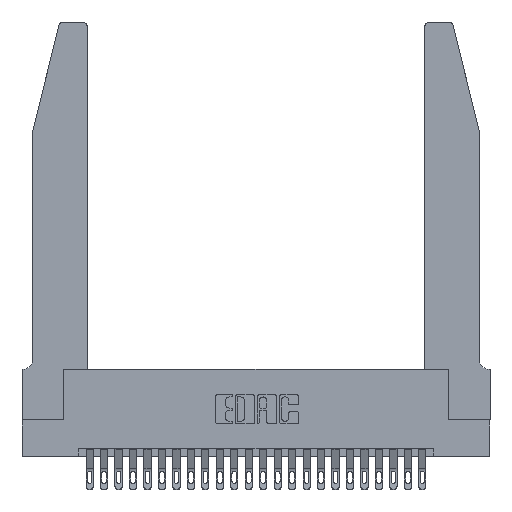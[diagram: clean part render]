
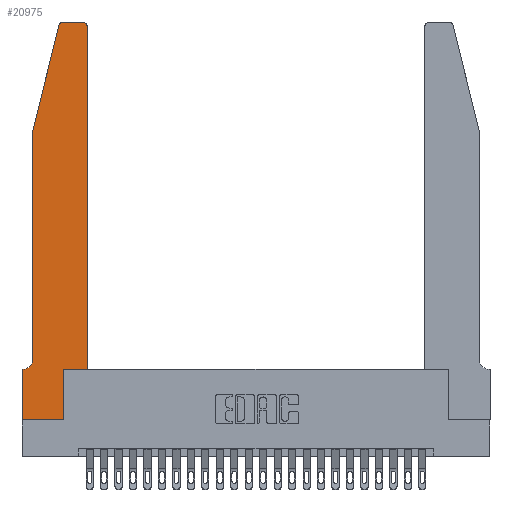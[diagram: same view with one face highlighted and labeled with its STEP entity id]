
A CAD part, top view. The second image highlights one B-rep face of the part: STEP entity #20975.
In plain terms, the highlighted planar face has unit normal (0, 0, 1).
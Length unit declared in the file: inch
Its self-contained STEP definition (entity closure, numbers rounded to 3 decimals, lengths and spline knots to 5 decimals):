
#20 = ORIENTED_EDGE ( 'NONE', *, *, #23290, .T. ) ;
#120 = CARTESIAN_POINT ( 'NONE',  ( 0.4505, 0.35, 0.37 ) ) ;
#456 = VECTOR ( 'NONE', #25401, 39.37008 ) ;
#581 = CARTESIAN_POINT ( 'NONE',  ( 0.4205, 2.72, 0.37 ) ) ;
#971 = DIRECTION ( 'NONE',  ( 0., -1., 0. ) ) ;
#1062 = VECTOR ( 'NONE', #4339, 39.37008 ) ;
#1375 = EDGE_LOOP ( 'NONE', ( #22535, #8584, #20704, #20, #17088, #1527, #10464, #9288, #26116, #14641, #14727, #2281 ) ) ;
#1527 = ORIENTED_EDGE ( 'NONE', *, *, #2855, .T. ) ;
#2210 = VECTOR ( 'NONE', #26248, 39.37008 ) ;
#2281 = ORIENTED_EDGE ( 'NONE', *, *, #10167, .T. ) ;
#2513 = CARTESIAN_POINT ( 'NONE',  ( 0., 0., 0.37 ) ) ;
#2573 = CARTESIAN_POINT ( 'NONE',  ( 0.4205, 2.75, 0.37 ) ) ;
#2686 = AXIS2_PLACEMENT_3D ( 'NONE', #581, #4804, #8976 ) ;
#2855 = EDGE_CURVE ( 'NONE', #21310, #16164, #23888, .T. ) ;
#3620 = CARTESIAN_POINT ( 'NONE',  ( 0.2605, 2.75, 0.37 ) ) ;
#4110 = DIRECTION ( 'NONE',  ( 0., 0., -1. ) ) ;
#4120 = DIRECTION ( 'NONE',  ( 0., 0., 1. ) ) ;
#4339 = DIRECTION ( 'NONE',  ( 1., 0., 0. ) ) ;
#4735 = PLANE ( 'NONE',  #20250 ) ;
#4804 = DIRECTION ( 'NONE',  ( 0., 0., 1. ) ) ;
#5156 = LINE ( 'NONE', #9257, #26128 ) ;
#6060 = VECTOR ( 'NONE', #12489, 39.37008 ) ;
#6342 = VERTEX_POINT ( 'NONE', #22943 ) ;
#6830 = CARTESIAN_POINT ( 'NONE',  ( 0.0055, 0.35, 0.37 ) ) ;
#6976 = DIRECTION ( 'NONE',  ( 0., -1., 0. ) ) ;
#7252 = CARTESIAN_POINT ( 'NONE',  ( 0.0755, 2., 0.37 ) ) ;
#7516 = CARTESIAN_POINT ( 'NONE',  ( 0.4505, 0.35, 0.37 ) ) ;
#7990 = VERTEX_POINT ( 'NONE', #2513 ) ;
#8584 = ORIENTED_EDGE ( 'NONE', *, *, #11825, .T. ) ;
#8708 = CIRCLE ( 'NONE', #20427, 0.07 ) ;
#8818 = VECTOR ( 'NONE', #17431, 39.37008 ) ;
#8968 = VERTEX_POINT ( 'NONE', #18181 ) ;
#8976 = DIRECTION ( 'NONE',  ( 1., 0., 0. ) ) ;
#9257 = CARTESIAN_POINT ( 'NONE',  ( 0.0755, 2., 0.37 ) ) ;
#9288 = ORIENTED_EDGE ( 'NONE', *, *, #12180, .T. ) ;
#9386 = FACE_OUTER_BOUND ( 'NONE', #1375, .T. ) ;
#9795 = DIRECTION ( 'NONE',  ( -1., 0., 0. ) ) ;
#9963 = LINE ( 'NONE', #120, #1062 ) ;
#10167 = EDGE_CURVE ( 'NONE', #8968, #24255, #17474, .T. ) ;
#10463 = VERTEX_POINT ( 'NONE', #10993 ) ;
#10464 = ORIENTED_EDGE ( 'NONE', *, *, #12732, .T. ) ;
#10773 = DIRECTION ( 'NONE',  ( 1., 0., 0. ) ) ;
#10993 = CARTESIAN_POINT ( 'NONE',  ( 0.4505, 0.35, 0.37 ) ) ;
#11049 = EDGE_CURVE ( 'NONE', #24833, #17696, #15502, .T. ) ;
#11497 = CARTESIAN_POINT ( 'NONE',  ( 0.0755, 2., 0.37 ) ) ;
#11825 = EDGE_CURVE ( 'NONE', #15092, #24833, #23747, .T. ) ;
#12180 = EDGE_CURVE ( 'NONE', #7990, #12327, #14835, .T. ) ;
#12327 = VERTEX_POINT ( 'NONE', #21972 ) ;
#12489 = DIRECTION ( 'NONE',  ( 0., 1., 0. ) ) ;
#12732 = EDGE_CURVE ( 'NONE', #16164, #7990, #16427, .T. ) ;
#13002 = CARTESIAN_POINT ( 'NONE',  ( 0., 0., 0.37 ) ) ;
#14641 = ORIENTED_EDGE ( 'NONE', *, *, #19251, .T. ) ;
#14671 = DIRECTION ( 'NONE',  ( 1., 0., 0. ) ) ;
#14727 = ORIENTED_EDGE ( 'NONE', *, *, #17780, .T. ) ;
#14788 = EDGE_CURVE ( 'NONE', #12327, #6342, #24489, .T. ) ;
#14835 = LINE ( 'NONE', #23316, #456 ) ;
#15092 = VERTEX_POINT ( 'NONE', #25351 ) ;
#15447 = VECTOR ( 'NONE', #9795, 39.37008 ) ;
#15502 = LINE ( 'NONE', #11497, #8818 ) ;
#15603 = CARTESIAN_POINT ( 'NONE',  ( 0.284, 2.72, 0.37 ) ) ;
#15745 = DIRECTION ( 'NONE',  ( 0., 1., 0. ) ) ;
#16164 = VERTEX_POINT ( 'NONE', #24701 ) ;
#16210 = AXIS2_PLACEMENT_3D ( 'NONE', #15603, #4120, #14671 ) ;
#16427 = LINE ( 'NONE', #13002, #24681 ) ;
#16743 = LINE ( 'NONE', #7516, #21543 ) ;
#16981 = CARTESIAN_POINT ( 'NONE',  ( 0.25487, 2.72718, 0.37 ) ) ;
#17088 = ORIENTED_EDGE ( 'NONE', *, *, #21775, .T. ) ;
#17431 = DIRECTION ( 'NONE',  ( -0.239, -0.971, 0. ) ) ;
#17474 = CIRCLE ( 'NONE', #2686, 0.03 ) ;
#17696 = VERTEX_POINT ( 'NONE', #7252 ) ;
#17780 = EDGE_CURVE ( 'NONE', #10463, #8968, #16743, .T. ) ;
#18181 = CARTESIAN_POINT ( 'NONE',  ( 0.4505, 2.72, 0.37 ) ) ;
#18197 = EDGE_CURVE ( 'NONE', #24255, #15092, #26252, .T. ) ;
#18326 = DIRECTION ( 'NONE',  ( -1., 0., 0. ) ) ;
#19251 = EDGE_CURVE ( 'NONE', #6342, #10463, #9963, .T. ) ;
#20009 = CARTESIAN_POINT ( 'NONE',  ( 0.0755, 0.42, 0.37 ) ) ;
#20250 = AXIS2_PLACEMENT_3D ( 'NONE', #20919, #23677, #10773 ) ;
#20298 = CARTESIAN_POINT ( 'NONE',  ( 0.0755, 0.35, 0.37 ) ) ;
#20427 = AXIS2_PLACEMENT_3D ( 'NONE', #22091, #4110, #18326 ) ;
#20704 = ORIENTED_EDGE ( 'NONE', *, *, #11049, .T. ) ;
#20919 = CARTESIAN_POINT ( 'NONE',  ( 0., 0.35, 0.37 ) ) ;
#20975 = ADVANCED_FACE ( 'NONE', ( #9386 ), #4735, .T. ) ;
#21310 = VERTEX_POINT ( 'NONE', #6830 ) ;
#21543 = VECTOR ( 'NONE', #15745, 39.37008 ) ;
#21714 = VERTEX_POINT ( 'NONE', #20009 ) ;
#21775 = EDGE_CURVE ( 'NONE', #21714, #21310, #8708, .T. ) ;
#21972 = CARTESIAN_POINT ( 'NONE',  ( 0.2865, 0., 0.37 ) ) ;
#22091 = CARTESIAN_POINT ( 'NONE',  ( 0.0055, 0.42, 0.37 ) ) ;
#22535 = ORIENTED_EDGE ( 'NONE', *, *, #18197, .T. ) ;
#22648 = CARTESIAN_POINT ( 'NONE',  ( 0.2865, 0.35, 0.37 ) ) ;
#22943 = CARTESIAN_POINT ( 'NONE',  ( 0.2865, 0.35, 0.37 ) ) ;
#23290 = EDGE_CURVE ( 'NONE', #17696, #21714, #5156, .T. ) ;
#23316 = CARTESIAN_POINT ( 'NONE',  ( 0., 0., 0.37 ) ) ;
#23677 = DIRECTION ( 'NONE',  ( 0., 0., 1. ) ) ;
#23747 = CIRCLE ( 'NONE', #16210, 0.03 ) ;
#23888 = LINE ( 'NONE', #20298, #2210 ) ;
#24255 = VERTEX_POINT ( 'NONE', #2573 ) ;
#24489 = LINE ( 'NONE', #22648, #6060 ) ;
#24681 = VECTOR ( 'NONE', #6976, 39.37008 ) ;
#24701 = CARTESIAN_POINT ( 'NONE',  ( 0., 0.35, 0.37 ) ) ;
#24833 = VERTEX_POINT ( 'NONE', #16981 ) ;
#25351 = CARTESIAN_POINT ( 'NONE',  ( 0.284, 2.75, 0.37 ) ) ;
#25401 = DIRECTION ( 'NONE',  ( 1., 0., 0. ) ) ;
#26116 = ORIENTED_EDGE ( 'NONE', *, *, #14788, .T. ) ;
#26128 = VECTOR ( 'NONE', #971, 39.37008 ) ;
#26248 = DIRECTION ( 'NONE',  ( -1., 0., 0. ) ) ;
#26252 = LINE ( 'NONE', #3620, #15447 ) ;
